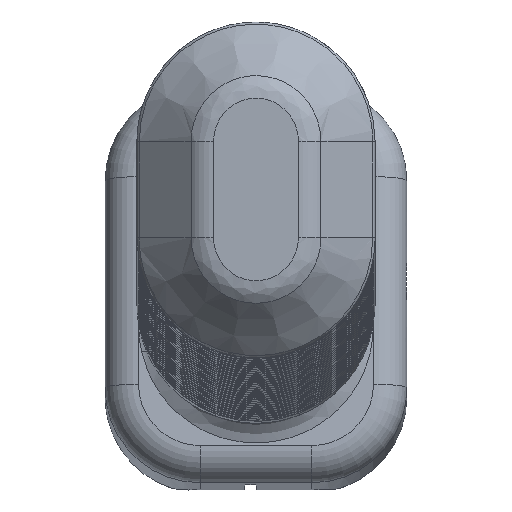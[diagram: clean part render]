
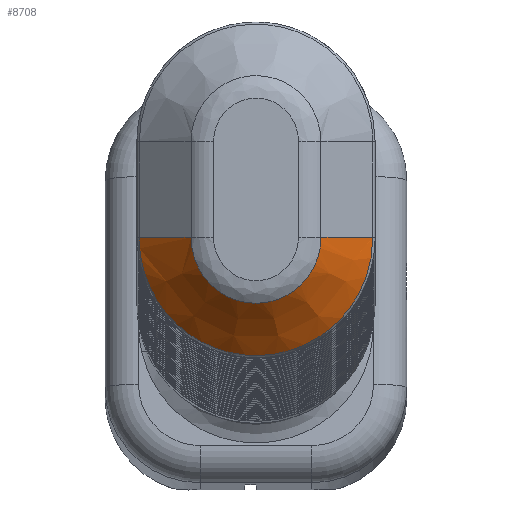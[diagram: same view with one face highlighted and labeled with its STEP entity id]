
A CAD part, front view. The second image highlights one B-rep face of the part: STEP entity #8708.
In plain terms, the highlighted free-form (B-spline) face has degree [3, 3] with [4, 10] control points.
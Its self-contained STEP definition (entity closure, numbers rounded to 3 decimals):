
#198=B_SPLINE_SURFACE_WITH_KNOTS('',3,3,((#29337,#29338,#29339,#29340,#29341,
#29342,#29343,#29344,#29345,#29346),(#29347,#29348,#29349,#29350,#29351,
#29352,#29353,#29354,#29355,#29356),(#29357,#29358,#29359,#29360,#29361,
#29362,#29363,#29364,#29365,#29366),(#29367,#29368,#29369,#29370,#29371,
#29372,#29373,#29374,#29375,#29376)),.UNSPECIFIED.,.F.,.F.,.F.,(4,4),(4,
1,1,1,1,1,1,4),(0.146,0.97),(-1.571,
-1.122,-0.673,-0.224,0.224,
0.673,1.122,1.571),.UNSPECIFIED.);
#934=B_SPLINE_CURVE_WITH_KNOTS('',3,(#29312,#29313,#29314,#29315,#29316,
#29317,#29318,#29319,#29320,#29321),.UNSPECIFIED.,.F.,.F.,(4,1,1,1,1,1,
1,4),(-1.696,-1.454,-1.212,-0.969,
-0.727,-0.485,-0.242,0.),
 .UNSPECIFIED.);
#936=B_SPLINE_CURVE_WITH_KNOTS('',3,(#29378,#29379,#29380,#29381),
 .UNSPECIFIED.,.F.,.F.,(4,4),(-0.005,0.),.UNSPECIFIED.);
#937=B_SPLINE_CURVE_WITH_KNOTS('',3,(#29383,#29384,#29385,#29386,#29387,
#29388,#29389,#29390,#29391,#29392),.UNSPECIFIED.,.F.,.F.,(4,1,1,1,1,1,
1,4),(0.,0.631,1.262,1.892,2.523,
3.154,3.785,4.416),.UNSPECIFIED.);
#938=B_SPLINE_CURVE_WITH_KNOTS('',3,(#29393,#29394,#29395,#29396),
 .UNSPECIFIED.,.F.,.F.,(4,4),(-0.005,0.),.UNSPECIFIED.);
#1872=FACE_OUTER_BOUND('',#2471,.T.);
#2471=EDGE_LOOP('',(#8044,#8045,#8046,#8047,#8048,#8049));
#2848=LINE('',#29122,#3225);
#2855=LINE('',#29224,#3232);
#3225=VECTOR('',#10672,10.);
#3232=VECTOR('',#10687,10.);
#4146=VERTEX_POINT('',#29118);
#4148=VERTEX_POINT('',#29121);
#4158=VERTEX_POINT('',#29221);
#4159=VERTEX_POINT('',#29223);
#4162=VERTEX_POINT('',#29377);
#4163=VERTEX_POINT('',#29382);
#5436=EDGE_CURVE('',#4148,#4146,#2848,.T.);
#5449=EDGE_CURVE('',#4159,#4158,#2855,.T.);
#5455=EDGE_CURVE('',#4148,#4158,#934,.T.);
#5459=EDGE_CURVE('',#4162,#4146,#936,.T.);
#5460=EDGE_CURVE('',#4163,#4162,#937,.T.);
#5461=EDGE_CURVE('',#4159,#4163,#938,.T.);
#8044=ORIENTED_EDGE('',*,*,#5459,.F.);
#8045=ORIENTED_EDGE('',*,*,#5460,.F.);
#8046=ORIENTED_EDGE('',*,*,#5461,.F.);
#8047=ORIENTED_EDGE('',*,*,#5449,.T.);
#8048=ORIENTED_EDGE('',*,*,#5455,.F.);
#8049=ORIENTED_EDGE('',*,*,#5436,.T.);
#8708=ADVANCED_FACE('',(#1872),#198,.T.);
#10672=DIRECTION('',(-0.707,0.707,0.));
#10687=DIRECTION('',(-0.707,-0.707,0.));
#29118=CARTESIAN_POINT('',(69.209,-101.293,44.749));
#29121=CARTESIAN_POINT('',(75.744,-107.828,44.749));
#29122=CARTESIAN_POINT('',(76.916,-109.,44.749));
#29221=CARTESIAN_POINT('',(92.087,-107.828,44.749));
#29223=CARTESIAN_POINT('',(98.623,-101.293,44.749));
#29224=CARTESIAN_POINT('',(98.916,-101.,44.749));
#29312=CARTESIAN_POINT('Ctrl Pts',(75.744,-107.828,44.749));
#29313=CARTESIAN_POINT('Ctrl Pts',(75.744,-107.828,43.531));
#29314=CARTESIAN_POINT('Ctrl Pts',(76.28,-107.828,41.095));
#29315=CARTESIAN_POINT('Ctrl Pts',(78.579,-107.828,38.102));
#29316=CARTESIAN_POINT('Ctrl Pts',(81.995,-107.828,36.395));
#29317=CARTESIAN_POINT('Ctrl Pts',(85.837,-107.828,36.393));
#29318=CARTESIAN_POINT('Ctrl Pts',(89.251,-107.828,38.103));
#29319=CARTESIAN_POINT('Ctrl Pts',(91.552,-107.828,41.094));
#29320=CARTESIAN_POINT('Ctrl Pts',(92.087,-107.828,43.531));
#29321=CARTESIAN_POINT('Ctrl Pts',(92.087,-107.828,44.749));
#29337=CARTESIAN_POINT('Ctrl Pts',(75.744,-107.828,44.749));
#29338=CARTESIAN_POINT('Ctrl Pts',(75.744,-107.828,43.502));
#29339=CARTESIAN_POINT('Ctrl Pts',(76.31,-107.828,41.009));
#29340=CARTESIAN_POINT('Ctrl Pts',(78.67,-107.828,38.032));
#29341=CARTESIAN_POINT('Ctrl Pts',(82.049,-107.828,36.395));
#29342=CARTESIAN_POINT('Ctrl Pts',(85.782,-107.828,36.397));
#29343=CARTESIAN_POINT('Ctrl Pts',(89.161,-107.828,38.031));
#29344=CARTESIAN_POINT('Ctrl Pts',(91.521,-107.828,41.009));
#29345=CARTESIAN_POINT('Ctrl Pts',(92.087,-107.828,43.502));
#29346=CARTESIAN_POINT('Ctrl Pts',(92.087,-107.828,44.749));
#29347=CARTESIAN_POINT('Ctrl Pts',(73.549,-105.633,44.749));
#29348=CARTESIAN_POINT('Ctrl Pts',(73.549,-105.633,43.176));
#29349=CARTESIAN_POINT('Ctrl Pts',(74.263,-105.633,40.031));
#29350=CARTESIAN_POINT('Ctrl Pts',(77.247,-105.633,36.263));
#29351=CARTESIAN_POINT('Ctrl Pts',(81.539,-105.633,34.182));
#29352=CARTESIAN_POINT('Ctrl Pts',(86.292,-105.633,34.184));
#29353=CARTESIAN_POINT('Ctrl Pts',(90.585,-105.633,36.262));
#29354=CARTESIAN_POINT('Ctrl Pts',(93.569,-105.633,40.032));
#29355=CARTESIAN_POINT('Ctrl Pts',(94.282,-105.633,43.176));
#29356=CARTESIAN_POINT('Ctrl Pts',(94.282,-105.633,44.749));
#29357=CARTESIAN_POINT('Ctrl Pts',(71.354,-103.438,44.749));
#29358=CARTESIAN_POINT('Ctrl Pts',(71.354,-103.438,42.85));
#29359=CARTESIAN_POINT('Ctrl Pts',(72.215,-103.438,39.054));
#29360=CARTESIAN_POINT('Ctrl Pts',(75.824,-103.438,34.494));
#29361=CARTESIAN_POINT('Ctrl Pts',(81.03,-103.438,31.968));
#29362=CARTESIAN_POINT('Ctrl Pts',(86.801,-103.438,31.971));
#29363=CARTESIAN_POINT('Ctrl Pts',(92.008,-103.438,34.492));
#29364=CARTESIAN_POINT('Ctrl Pts',(95.617,-103.438,39.054));
#29365=CARTESIAN_POINT('Ctrl Pts',(96.477,-103.438,42.85));
#29366=CARTESIAN_POINT('Ctrl Pts',(96.477,-103.438,44.749));
#29367=CARTESIAN_POINT('Ctrl Pts',(69.159,-101.243,44.749));
#29368=CARTESIAN_POINT('Ctrl Pts',(69.159,-101.243,42.524));
#29369=CARTESIAN_POINT('Ctrl Pts',(70.167,-101.243,38.076));
#29370=CARTESIAN_POINT('Ctrl Pts',(74.401,-101.243,32.725));
#29371=CARTESIAN_POINT('Ctrl Pts',(80.52,-101.243,29.754));
#29372=CARTESIAN_POINT('Ctrl Pts',(87.311,-101.243,29.758));
#29373=CARTESIAN_POINT('Ctrl Pts',(93.431,-101.243,32.723));
#29374=CARTESIAN_POINT('Ctrl Pts',(97.664,-101.243,38.076));
#29375=CARTESIAN_POINT('Ctrl Pts',(98.672,-101.243,42.524));
#29376=CARTESIAN_POINT('Ctrl Pts',(98.672,-101.243,44.749));
#29377=CARTESIAN_POINT('',(69.209,-101.293,44.695));
#29378=CARTESIAN_POINT('Ctrl Pts',(69.209,-101.293,44.695));
#29379=CARTESIAN_POINT('Ctrl Pts',(69.209,-101.293,44.713));
#29380=CARTESIAN_POINT('Ctrl Pts',(69.209,-101.293,44.731));
#29381=CARTESIAN_POINT('Ctrl Pts',(69.209,-101.293,44.749));
#29382=CARTESIAN_POINT('',(98.623,-101.293,44.695));
#29383=CARTESIAN_POINT('Ctrl Pts',(98.623,-101.293,44.695));
#29384=CARTESIAN_POINT('Ctrl Pts',(98.622,-101.285,42.488));
#29385=CARTESIAN_POINT('Ctrl Pts',(97.627,-101.27,38.075));
#29386=CARTESIAN_POINT('Ctrl Pts',(93.428,-101.253,32.738));
#29387=CARTESIAN_POINT('Ctrl Pts',(87.317,-101.243,29.754));
#29388=CARTESIAN_POINT('Ctrl Pts',(80.515,-101.243,29.758));
#29389=CARTESIAN_POINT('Ctrl Pts',(74.403,-101.253,32.736));
#29390=CARTESIAN_POINT('Ctrl Pts',(70.204,-101.27,38.076));
#29391=CARTESIAN_POINT('Ctrl Pts',(69.209,-101.285,42.488));
#29392=CARTESIAN_POINT('Ctrl Pts',(69.209,-101.293,44.695));
#29393=CARTESIAN_POINT('Ctrl Pts',(98.623,-101.293,44.749));
#29394=CARTESIAN_POINT('Ctrl Pts',(98.623,-101.293,44.731));
#29395=CARTESIAN_POINT('Ctrl Pts',(98.623,-101.293,44.713));
#29396=CARTESIAN_POINT('Ctrl Pts',(98.623,-101.293,44.695));
